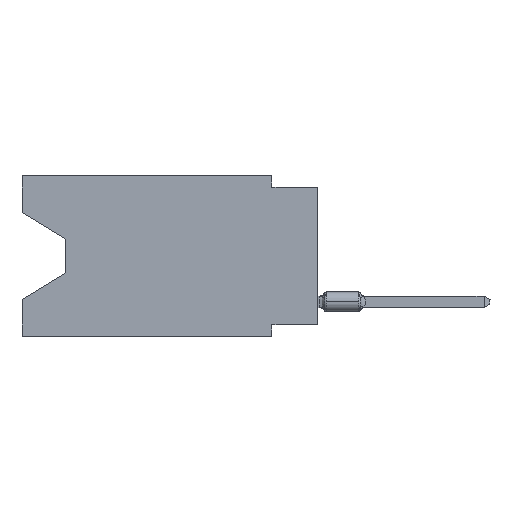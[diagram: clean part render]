
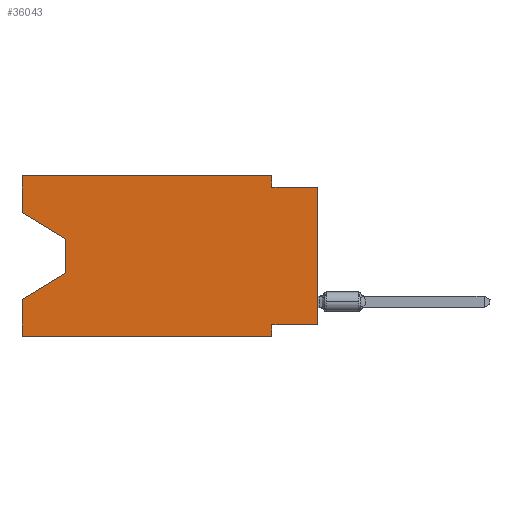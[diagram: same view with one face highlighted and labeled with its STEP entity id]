
A CAD part, left-side view. The second image highlights one B-rep face of the part: STEP entity #36043.
In plain terms, the highlighted planar face has unit normal (-1, 0, 0).
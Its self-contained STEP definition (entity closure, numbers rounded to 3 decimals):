
#123 = CARTESIAN_POINT ( 'NONE',  ( 0., 2.54, -8.255 ) ) ;
#271 = VERTEX_POINT ( 'NONE', #14169 ) ;
#406 = ORIENTED_EDGE ( 'NONE', *, *, #4783, .F. ) ;
#1160 = CARTESIAN_POINT ( 'NONE',  ( 0., 13.97, -3.505 ) ) ;
#1458 = ORIENTED_EDGE ( 'NONE', *, *, #6654, .T. ) ;
#2458 = CARTESIAN_POINT ( 'NONE',  ( 0., 16.383, -8.89 ) ) ;
#3631 = LINE ( 'NONE', #31717, #44878 ) ;
#3714 = CARTESIAN_POINT ( 'NONE',  ( 0., 2.54, 0. ) ) ;
#4666 = ORIENTED_EDGE ( 'NONE', *, *, #42130, .F. ) ;
#4783 = EDGE_CURVE ( 'NONE', #9235, #17758, #32734, .T. ) ;
#4958 = PLANE ( 'NONE',  #38916 ) ;
#5345 = CARTESIAN_POINT ( 'NONE',  ( 0., 16.383, -2.038 ) ) ;
#5490 = LINE ( 'NONE', #30820, #32546 ) ;
#6109 = VECTOR ( 'NONE', #29275, 1000. ) ;
#6654 = EDGE_CURVE ( 'NONE', #13108, #38117, #23071, .T. ) ;
#6719 = VERTEX_POINT ( 'NONE', #123 ) ;
#8663 = DIRECTION ( 'NONE',  ( 0., 0., 1. ) ) ;
#9235 = VERTEX_POINT ( 'NONE', #27057 ) ;
#9377 = CARTESIAN_POINT ( 'NONE',  ( 0., 0., 0. ) ) ;
#9668 = EDGE_CURVE ( 'NONE', #34610, #271, #29527, .T. ) ;
#10226 = ORIENTED_EDGE ( 'NONE', *, *, #26068, .F. ) ;
#10710 = CARTESIAN_POINT ( 'NONE',  ( 0., 0., -8.255 ) ) ;
#11463 = CARTESIAN_POINT ( 'NONE',  ( 0., 2.54, -8.89 ) ) ;
#12840 = CARTESIAN_POINT ( 'NONE',  ( 0., 16.383, 0. ) ) ;
#12875 = EDGE_CURVE ( 'NONE', #26151, #9235, #29449, .T. ) ;
#13108 = VERTEX_POINT ( 'NONE', #25587 ) ;
#14169 = CARTESIAN_POINT ( 'NONE',  ( 0., 13.97, -5.385 ) ) ;
#16733 = VECTOR ( 'NONE', #34710, 1000. ) ;
#16950 = EDGE_CURVE ( 'NONE', #30097, #36984, #19962, .T. ) ;
#17326 = VECTOR ( 'NONE', #22680, 1000. ) ;
#17758 = VERTEX_POINT ( 'NONE', #30289 ) ;
#18663 = CARTESIAN_POINT ( 'NONE',  ( 0., 16.383, 0. ) ) ;
#19962 = LINE ( 'NONE', #40977, #32639 ) ;
#20077 = EDGE_CURVE ( 'NONE', #17758, #44409, #28363, .T. ) ;
#20407 = VECTOR ( 'NONE', #42305, 1000. ) ;
#20989 = DIRECTION ( 'NONE',  ( 0., 1., 0. ) ) ;
#21147 = ORIENTED_EDGE ( 'NONE', *, *, #12875, .F. ) ;
#22095 = FACE_OUTER_BOUND ( 'NONE', #25486, .T. ) ;
#22680 = DIRECTION ( 'NONE',  ( 0., -1., 0. ) ) ;
#23071 = LINE ( 'NONE', #9377, #27611 ) ;
#23443 = VECTOR ( 'NONE', #26092, 1000. ) ;
#24289 = DIRECTION ( 'NONE',  ( 0., 0., 1. ) ) ;
#25486 = EDGE_LOOP ( 'NONE', ( #40112, #35459, #40769, #41468, #38842, #40250, #10226, #1458, #4666, #32599, #406, #21147 ) ) ;
#25587 = CARTESIAN_POINT ( 'NONE',  ( 0., 0., -8.255 ) ) ;
#25962 = EDGE_CURVE ( 'NONE', #30097, #34063, #5490, .T. ) ;
#26068 = EDGE_CURVE ( 'NONE', #13108, #6719, #27615, .T. ) ;
#26092 = DIRECTION ( 'NONE',  ( 0., 0., -1. ) ) ;
#26151 = VERTEX_POINT ( 'NONE', #28529 ) ;
#26349 = DIRECTION ( 'NONE',  ( 0., -0.855, -0.519 ) ) ;
#27057 = CARTESIAN_POINT ( 'NONE',  ( 0., 16.383, 0. ) ) ;
#27149 = CARTESIAN_POINT ( 'NONE',  ( 0., 16.383, -6.852 ) ) ;
#27611 = VECTOR ( 'NONE', #37243, 1000. ) ;
#27615 = LINE ( 'NONE', #10710, #36951 ) ;
#28363 = LINE ( 'NONE', #3714, #20407 ) ;
#28529 = CARTESIAN_POINT ( 'NONE',  ( 0., 16.383, -2.038 ) ) ;
#29275 = DIRECTION ( 'NONE',  ( 0., 0., -1. ) ) ;
#29449 = LINE ( 'NONE', #43831, #35934 ) ;
#29527 = LINE ( 'NONE', #43461, #23443 ) ;
#30097 = VERTEX_POINT ( 'NONE', #2458 ) ;
#30132 = VECTOR ( 'NONE', #26349, 1000. ) ;
#30230 = CARTESIAN_POINT ( 'NONE',  ( 0., 0., -0.635 ) ) ;
#30289 = CARTESIAN_POINT ( 'NONE',  ( 0., 2.54, 0. ) ) ;
#30820 = CARTESIAN_POINT ( 'NONE',  ( 0., 16.383, -8.89 ) ) ;
#31033 = DIRECTION ( 'NONE',  ( 0., 0.855, -0.519 ) ) ;
#31650 = EDGE_CURVE ( 'NONE', #271, #36984, #3631, .T. ) ;
#31717 = CARTESIAN_POINT ( 'NONE',  ( 0., 13.97, -5.385 ) ) ;
#32546 = VECTOR ( 'NONE', #44760, 1000. ) ;
#32599 = ORIENTED_EDGE ( 'NONE', *, *, #20077, .F. ) ;
#32639 = VECTOR ( 'NONE', #24289, 1000. ) ;
#32734 = LINE ( 'NONE', #12840, #17326 ) ;
#34063 = VERTEX_POINT ( 'NONE', #38904 ) ;
#34491 = CARTESIAN_POINT ( 'NONE',  ( 0., 0., -0.635 ) ) ;
#34610 = VERTEX_POINT ( 'NONE', #1160 ) ;
#34710 = DIRECTION ( 'NONE',  ( 0., -1., 0. ) ) ;
#35459 = ORIENTED_EDGE ( 'NONE', *, *, #9668, .T. ) ;
#35934 = VECTOR ( 'NONE', #8663, 1000. ) ;
#36026 = DIRECTION ( 'NONE',  ( 0., 0., -1. ) ) ;
#36043 = ADVANCED_FACE ( 'NONE', ( #22095 ), #4958, .F. ) ;
#36951 = VECTOR ( 'NONE', #20989, 1000. ) ;
#36984 = VERTEX_POINT ( 'NONE', #27149 ) ;
#37243 = DIRECTION ( 'NONE',  ( 0., 0., 1. ) ) ;
#38117 = VERTEX_POINT ( 'NONE', #30230 ) ;
#38842 = ORIENTED_EDGE ( 'NONE', *, *, #25962, .T. ) ;
#38904 = CARTESIAN_POINT ( 'NONE',  ( 0., 2.54, -8.89 ) ) ;
#38916 = AXIS2_PLACEMENT_3D ( 'NONE', #18663, #40133, #36026 ) ;
#39883 = EDGE_CURVE ( 'NONE', #26151, #34610, #40507, .T. ) ;
#40112 = ORIENTED_EDGE ( 'NONE', *, *, #39883, .T. ) ;
#40133 = DIRECTION ( 'NONE',  ( 1., 0., 0. ) ) ;
#40250 = ORIENTED_EDGE ( 'NONE', *, *, #41810, .F. ) ;
#40507 = LINE ( 'NONE', #5345, #30132 ) ;
#40769 = ORIENTED_EDGE ( 'NONE', *, *, #31650, .T. ) ;
#40977 = CARTESIAN_POINT ( 'NONE',  ( 0., 16.383, 0. ) ) ;
#41468 = ORIENTED_EDGE ( 'NONE', *, *, #16950, .F. ) ;
#41810 = EDGE_CURVE ( 'NONE', #6719, #34063, #42760, .T. ) ;
#42130 = EDGE_CURVE ( 'NONE', #44409, #38117, #42484, .T. ) ;
#42305 = DIRECTION ( 'NONE',  ( 0., 0., -1. ) ) ;
#42484 = LINE ( 'NONE', #34491, #16733 ) ;
#42760 = LINE ( 'NONE', #11463, #6109 ) ;
#43461 = CARTESIAN_POINT ( 'NONE',  ( 0., 13.97, -3.505 ) ) ;
#43831 = CARTESIAN_POINT ( 'NONE',  ( 0., 16.383, 0. ) ) ;
#44409 = VERTEX_POINT ( 'NONE', #45118 ) ;
#44760 = DIRECTION ( 'NONE',  ( 0., -1., 0. ) ) ;
#44878 = VECTOR ( 'NONE', #31033, 1000. ) ;
#45118 = CARTESIAN_POINT ( 'NONE',  ( 0., 2.54, -0.635 ) ) ;
